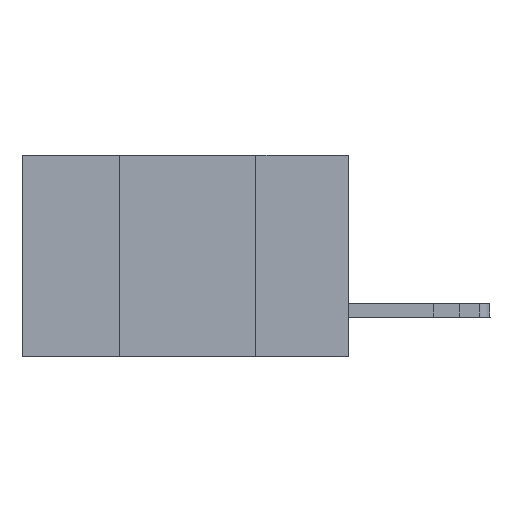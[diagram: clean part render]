
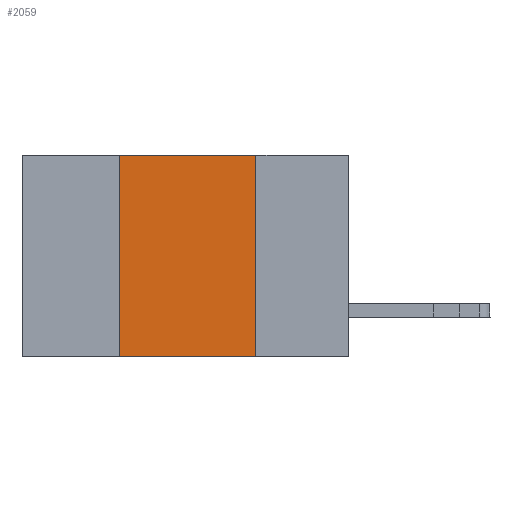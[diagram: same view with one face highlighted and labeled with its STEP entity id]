
A CAD part, left-side view. The second image highlights one B-rep face of the part: STEP entity #2059.
In plain terms, the highlighted planar face has unit normal (-1, 0, 0).
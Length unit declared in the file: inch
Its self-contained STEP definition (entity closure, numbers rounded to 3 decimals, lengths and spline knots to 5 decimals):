
#348 = ORIENTED_EDGE ( 'NONE', *, *, #17806, .T. ) ;
#677 = LINE ( 'NONE', #26237, #994 ) ;
#875 = CARTESIAN_POINT ( 'NONE',  ( 0., 0.42, -0.37 ) ) ;
#994 = VECTOR ( 'NONE', #15270, 39.37008 ) ;
#1256 = LINE ( 'NONE', #5688, #8821 ) ;
#1905 = ORIENTED_EDGE ( 'NONE', *, *, #22514, .F. ) ;
#2056 = DIRECTION ( 'NONE',  ( 0., 0., -1. ) ) ;
#2059 = ADVANCED_FACE ( 'NONE', ( #25461 ), #4477, .F. ) ;
#3818 = CARTESIAN_POINT ( 'NONE',  ( 0., 0.42, 0. ) ) ;
#4477 = PLANE ( 'NONE',  #23852 ) ;
#4695 = VERTEX_POINT ( 'NONE', #19369 ) ;
#4826 = ORIENTED_EDGE ( 'NONE', *, *, #15178, .F. ) ;
#5288 = CARTESIAN_POINT ( 'NONE',  ( 0., 0.17, 0. ) ) ;
#5688 = CARTESIAN_POINT ( 'NONE',  ( 0., 0.6, 0. ) ) ;
#8176 = DIRECTION ( 'NONE',  ( 0., -1., 0. ) ) ;
#8821 = VECTOR ( 'NONE', #8176, 39.37008 ) ;
#10318 = DIRECTION ( 'NONE',  ( 0., 0., 1. ) ) ;
#11302 = LINE ( 'NONE', #19186, #26342 ) ;
#14907 = VERTEX_POINT ( 'NONE', #5288 ) ;
#15178 = EDGE_CURVE ( 'NONE', #14907, #4695, #19479, .T. ) ;
#15194 = DIRECTION ( 'NONE',  ( 1., 0., 0. ) ) ;
#15270 = DIRECTION ( 'NONE',  ( 0., -1., 0. ) ) ;
#17625 = DIRECTION ( 'NONE',  ( 0., 0., -1. ) ) ;
#17804 = ORIENTED_EDGE ( 'NONE', *, *, #26229, .F. ) ;
#17806 = EDGE_CURVE ( 'NONE', #18697, #4695, #677, .T. ) ;
#18697 = VERTEX_POINT ( 'NONE', #875 ) ;
#18962 = VERTEX_POINT ( 'NONE', #3818 ) ;
#19186 = CARTESIAN_POINT ( 'NONE',  ( 0., 0.42, 0. ) ) ;
#19369 = CARTESIAN_POINT ( 'NONE',  ( 0., 0.17, -0.37 ) ) ;
#19479 = LINE ( 'NONE', #21252, #22794 ) ;
#21252 = CARTESIAN_POINT ( 'NONE',  ( 0., 0.17, 0. ) ) ;
#21922 = CARTESIAN_POINT ( 'NONE',  ( 0., 0.6, 0. ) ) ;
#22514 = EDGE_CURVE ( 'NONE', #18962, #14907, #1256, .T. ) ;
#22794 = VECTOR ( 'NONE', #2056, 39.37008 ) ;
#23852 = AXIS2_PLACEMENT_3D ( 'NONE', #21922, #15194, #17625 ) ;
#24643 = EDGE_LOOP ( 'NONE', ( #4826, #1905, #17804, #348 ) ) ;
#25461 = FACE_OUTER_BOUND ( 'NONE', #24643, .T. ) ;
#26229 = EDGE_CURVE ( 'NONE', #18697, #18962, #11302, .T. ) ;
#26237 = CARTESIAN_POINT ( 'NONE',  ( 0., 0.6, -0.37 ) ) ;
#26342 = VECTOR ( 'NONE', #10318, 39.37008 ) ;
